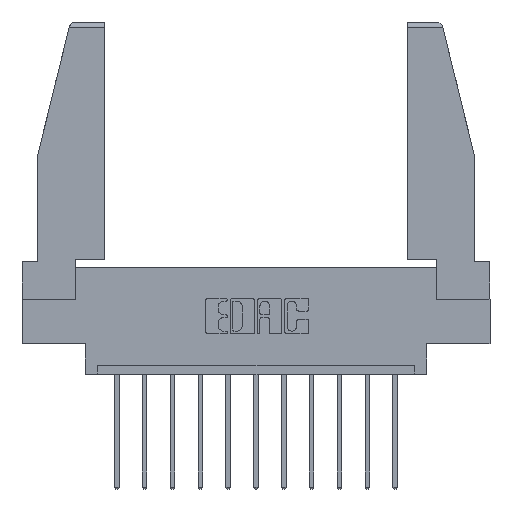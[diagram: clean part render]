
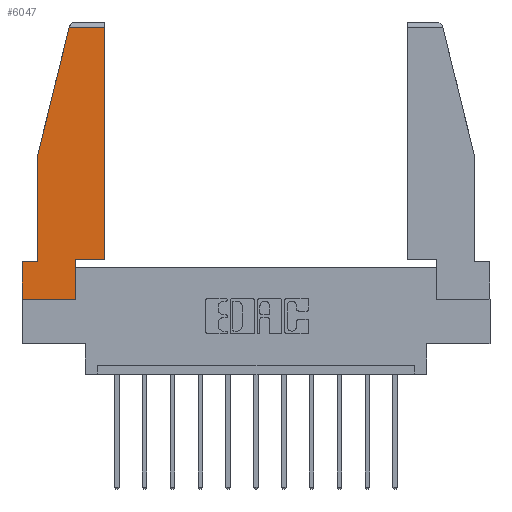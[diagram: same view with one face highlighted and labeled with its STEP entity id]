
A CAD part, top view. The second image highlights one B-rep face of the part: STEP entity #6047.
In plain terms, the highlighted planar face has unit normal (0, 0, 1).
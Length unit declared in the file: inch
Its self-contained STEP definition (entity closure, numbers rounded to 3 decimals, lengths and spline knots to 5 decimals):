
#32 = DIRECTION ( 'NONE',  ( 0., -1., 0. ) ) ;
#76 = ORIENTED_EDGE ( 'NONE', *, *, #2502, .T. ) ;
#84 = ORIENTED_EDGE ( 'NONE', *, *, #14211, .T. ) ;
#259 = VERTEX_POINT ( 'NONE', #4650 ) ;
#605 = VECTOR ( 'NONE', #12732, 39.37008 ) ;
#621 = VERTEX_POINT ( 'NONE', #5238 ) ;
#675 = CARTESIAN_POINT ( 'NONE',  ( 0.297, 0., 0. ) ) ;
#800 = DIRECTION ( 'NONE',  ( 1., 0., 0. ) ) ;
#810 = DIRECTION ( 'NONE',  ( 1., 0., 0. ) ) ;
#879 = VERTEX_POINT ( 'NONE', #2969 ) ;
#979 = VECTOR ( 'NONE', #3597, 39.37008 ) ;
#1065 = EDGE_CURVE ( 'NONE', #14385, #259, #11802, .T. ) ;
#1120 = ORIENTED_EDGE ( 'NONE', *, *, #7684, .T. ) ;
#1141 = VECTOR ( 'NONE', #32, 39.37008 ) ;
#1512 = DIRECTION ( 'NONE',  ( 0., 1., 0. ) ) ;
#1629 = DIRECTION ( 'NONE',  ( 0., -1., 0. ) ) ;
#1703 = VECTOR ( 'NONE', #4411, 39.37008 ) ;
#1726 = CARTESIAN_POINT ( 'NONE',  ( 0., 0.21, 0. ) ) ;
#1806 = ORIENTED_EDGE ( 'NONE', *, *, #1065, .T. ) ;
#1952 = EDGE_CURVE ( 'NONE', #10785, #2960, #14575, .T. ) ;
#1961 = AXIS2_PLACEMENT_3D ( 'NONE', #10953, #7553, #810 ) ;
#2502 = EDGE_CURVE ( 'NONE', #621, #10785, #7205, .T. ) ;
#2736 = ORIENTED_EDGE ( 'NONE', *, *, #12521, .T. ) ;
#2853 = VECTOR ( 'NONE', #11999, 39.37008 ) ;
#2960 = VERTEX_POINT ( 'NONE', #8472 ) ;
#2969 = CARTESIAN_POINT ( 'NONE',  ( 0.461, 0.223, 0. ) ) ;
#3010 = EDGE_CURVE ( 'NONE', #14273, #13667, #7386, .T. ) ;
#3597 = DIRECTION ( 'NONE',  ( -0.239, -0.971, 0. ) ) ;
#4036 = CARTESIAN_POINT ( 'NONE',  ( 0., 0.21, 0. ) ) ;
#4187 = LINE ( 'NONE', #12419, #1141 ) ;
#4411 = DIRECTION ( 'NONE',  ( 1., 0., 0. ) ) ;
#4650 = CARTESIAN_POINT ( 'NONE',  ( 0., 0.21, 0. ) ) ;
#5196 = PLANE ( 'NONE',  #1961 ) ;
#5200 = EDGE_LOOP ( 'NONE', ( #11872, #76, #10006, #1120, #1806, #84, #5668, #2736, #13708 ) ) ;
#5238 = CARTESIAN_POINT ( 'NONE',  ( 0.461, 1.52, 0. ) ) ;
#5668 = ORIENTED_EDGE ( 'NONE', *, *, #3010, .T. ) ;
#6047 = ADVANCED_FACE ( 'NONE', ( #6417 ), #5196, .T. ) ;
#6417 = FACE_OUTER_BOUND ( 'NONE', #5200, .T. ) ;
#7205 = LINE ( 'NONE', #12883, #605 ) ;
#7385 = VECTOR ( 'NONE', #1629, 39.37008 ) ;
#7386 = LINE ( 'NONE', #10898, #12044 ) ;
#7427 = LINE ( 'NONE', #11264, #1703 ) ;
#7553 = DIRECTION ( 'NONE',  ( 0., 0., 1. ) ) ;
#7684 = EDGE_CURVE ( 'NONE', #2960, #14385, #4187, .T. ) ;
#8268 = CARTESIAN_POINT ( 'NONE',  ( 0.271, 1.55, 0. ) ) ;
#8472 = CARTESIAN_POINT ( 'NONE',  ( 0.086, 0.8, 0. ) ) ;
#8489 = CARTESIAN_POINT ( 'NONE',  ( 0.2636, 1.52, 0. ) ) ;
#8706 = VECTOR ( 'NONE', #14267, 39.37008 ) ;
#8840 = CARTESIAN_POINT ( 'NONE',  ( 0.086, 0.21, 0. ) ) ;
#10006 = ORIENTED_EDGE ( 'NONE', *, *, #1952, .T. ) ;
#10420 = LINE ( 'NONE', #1726, #7385 ) ;
#10465 = VERTEX_POINT ( 'NONE', #11569 ) ;
#10785 = VERTEX_POINT ( 'NONE', #8489 ) ;
#10898 = CARTESIAN_POINT ( 'NONE',  ( 0., 0., 0. ) ) ;
#10953 = CARTESIAN_POINT ( 'NONE',  ( 0., 0., 0. ) ) ;
#11264 = CARTESIAN_POINT ( 'NONE',  ( 0.297, 0.223, 0. ) ) ;
#11569 = CARTESIAN_POINT ( 'NONE',  ( 0.297, 0.223, 0. ) ) ;
#11719 = CARTESIAN_POINT ( 'NONE',  ( 0.461, 0.223, 0. ) ) ;
#11802 = LINE ( 'NONE', #4036, #2853 ) ;
#11872 = ORIENTED_EDGE ( 'NONE', *, *, #14749, .T. ) ;
#11999 = DIRECTION ( 'NONE',  ( -1., 0., 0. ) ) ;
#12027 = LINE ( 'NONE', #11719, #14685 ) ;
#12044 = VECTOR ( 'NONE', #800, 39.37008 ) ;
#12102 = LINE ( 'NONE', #675, #8706 ) ;
#12419 = CARTESIAN_POINT ( 'NONE',  ( 0.086, 0.8, 0. ) ) ;
#12521 = EDGE_CURVE ( 'NONE', #13667, #10465, #12102, .T. ) ;
#12685 = EDGE_CURVE ( 'NONE', #10465, #879, #7427, .T. ) ;
#12732 = DIRECTION ( 'NONE',  ( -1., 0., 0. ) ) ;
#12883 = CARTESIAN_POINT ( 'NONE',  ( 0., 1.52, 0. ) ) ;
#13122 = CARTESIAN_POINT ( 'NONE',  ( 0., 0., 0. ) ) ;
#13382 = CARTESIAN_POINT ( 'NONE',  ( 0.297, 0., 0. ) ) ;
#13667 = VERTEX_POINT ( 'NONE', #13382 ) ;
#13708 = ORIENTED_EDGE ( 'NONE', *, *, #12685, .T. ) ;
#14211 = EDGE_CURVE ( 'NONE', #259, #14273, #10420, .T. ) ;
#14267 = DIRECTION ( 'NONE',  ( 0., 1., 0. ) ) ;
#14273 = VERTEX_POINT ( 'NONE', #13122 ) ;
#14385 = VERTEX_POINT ( 'NONE', #8840 ) ;
#14575 = LINE ( 'NONE', #8268, #979 ) ;
#14685 = VECTOR ( 'NONE', #1512, 39.37008 ) ;
#14749 = EDGE_CURVE ( 'NONE', #879, #621, #12027, .T. ) ;
